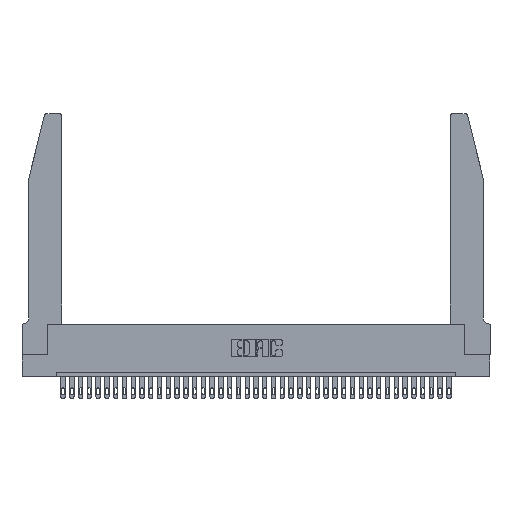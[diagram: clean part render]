
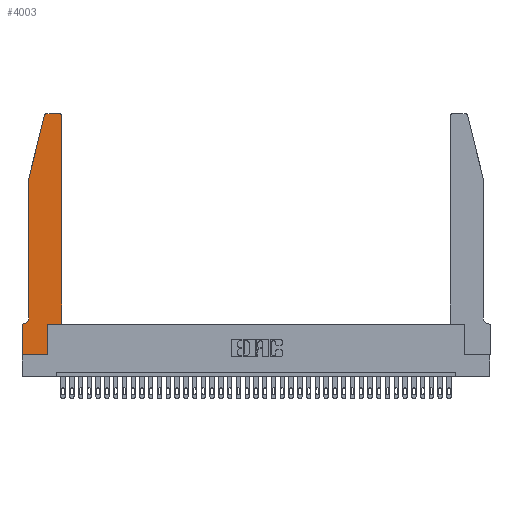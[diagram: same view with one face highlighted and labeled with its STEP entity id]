
A CAD part, top view. The second image highlights one B-rep face of the part: STEP entity #4003.
In plain terms, the highlighted planar face has unit normal (0, 0, 1).
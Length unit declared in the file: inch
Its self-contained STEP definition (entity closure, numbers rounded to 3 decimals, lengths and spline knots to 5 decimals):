
#663 = EDGE_CURVE ( 'NONE', #30695, #31927, #8686, .T. ) ;
#810 = FACE_OUTER_BOUND ( 'NONE', #34364, .T. ) ;
#1058 = ORIENTED_EDGE ( 'NONE', *, *, #20345, .T. ) ;
#1081 = CARTESIAN_POINT ( 'NONE',  ( 0.4505, 2.72, 0.37 ) ) ;
#1657 = CARTESIAN_POINT ( 'NONE',  ( 0.4505, 0.35, 0.37 ) ) ;
#1691 = DIRECTION ( 'NONE',  ( 1., 0., 0. ) ) ;
#2081 = VECTOR ( 'NONE', #19001, 39.37008 ) ;
#2313 = VERTEX_POINT ( 'NONE', #20618 ) ;
#2601 = CIRCLE ( 'NONE', #14978, 0.03 ) ;
#2822 = EDGE_CURVE ( 'NONE', #29767, #29390, #4620, .T. ) ;
#3044 = VECTOR ( 'NONE', #21404, 39.37008 ) ;
#3677 = AXIS2_PLACEMENT_3D ( 'NONE', #16455, #25176, #33824 ) ;
#3900 = CIRCLE ( 'NONE', #3677, 0.03 ) ;
#4003 = ADVANCED_FACE ( 'NONE', ( #810 ), #4917, .T. ) ;
#4620 = LINE ( 'NONE', #9189, #35060 ) ;
#4917 = PLANE ( 'NONE',  #35814 ) ;
#5079 = VECTOR ( 'NONE', #15449, 39.37008 ) ;
#5183 = DIRECTION ( 'NONE',  ( 0., -1., 0. ) ) ;
#5932 = VECTOR ( 'NONE', #5183, 39.37008 ) ;
#6243 = EDGE_CURVE ( 'NONE', #29390, #14842, #16583, .T. ) ;
#6562 = CARTESIAN_POINT ( 'NONE',  ( 0.284, 2.75, 0.37 ) ) ;
#6778 = ORIENTED_EDGE ( 'NONE', *, *, #32845, .T. ) ;
#6793 = VECTOR ( 'NONE', #25274, 39.37008 ) ;
#6817 = ORIENTED_EDGE ( 'NONE', *, *, #2822, .T. ) ;
#7348 = DIRECTION ( 'NONE',  ( -1., 0., 0. ) ) ;
#7484 = CARTESIAN_POINT ( 'NONE',  ( 0.2605, 2.75, 0.37 ) ) ;
#7898 = DIRECTION ( 'NONE',  ( 0., 0., 1. ) ) ;
#8686 = LINE ( 'NONE', #1657, #10536 ) ;
#9189 = CARTESIAN_POINT ( 'NONE',  ( 0.0755, 2., 0.37 ) ) ;
#9199 = VERTEX_POINT ( 'NONE', #22762 ) ;
#9320 = CARTESIAN_POINT ( 'NONE',  ( 0.0755, 0.35, 0.37 ) ) ;
#10508 = VERTEX_POINT ( 'NONE', #23438 ) ;
#10536 = VECTOR ( 'NONE', #34135, 39.37008 ) ;
#10606 = CARTESIAN_POINT ( 'NONE',  ( 0.4205, 2.75, 0.37 ) ) ;
#10871 = CARTESIAN_POINT ( 'NONE',  ( 0., 0.35, 0.37 ) ) ;
#12370 = CARTESIAN_POINT ( 'NONE',  ( 0.0755, 0.42, 0.37 ) ) ;
#13164 = CARTESIAN_POINT ( 'NONE',  ( 0., 0., 0.37 ) ) ;
#13927 = CARTESIAN_POINT ( 'NONE',  ( 0.4505, 0.35, 0.37 ) ) ;
#14587 = ORIENTED_EDGE ( 'NONE', *, *, #22725, .T. ) ;
#14842 = VERTEX_POINT ( 'NONE', #12370 ) ;
#14978 = AXIS2_PLACEMENT_3D ( 'NONE', #21487, #36275, #33474 ) ;
#15449 = DIRECTION ( 'NONE',  ( 1., 0., 0. ) ) ;
#16076 = CARTESIAN_POINT ( 'NONE',  ( 0., 0., 0.37 ) ) ;
#16382 = ORIENTED_EDGE ( 'NONE', *, *, #663, .T. ) ;
#16436 = CARTESIAN_POINT ( 'NONE',  ( 0.0055, 0.42, 0.37 ) ) ;
#16455 = CARTESIAN_POINT ( 'NONE',  ( 0.284, 2.72, 0.37 ) ) ;
#16583 = LINE ( 'NONE', #36699, #5932 ) ;
#16997 = LINE ( 'NONE', #7484, #25711 ) ;
#17065 = LINE ( 'NONE', #21554, #5079 ) ;
#17126 = VERTEX_POINT ( 'NONE', #13164 ) ;
#17236 = ORIENTED_EDGE ( 'NONE', *, *, #33155, .T. ) ;
#18017 = CARTESIAN_POINT ( 'NONE',  ( 0.2865, 0.35, 0.37 ) ) ;
#18339 = DIRECTION ( 'NONE',  ( -0.239, -0.971, 0. ) ) ;
#19001 = DIRECTION ( 'NONE',  ( 0., -1., 0. ) ) ;
#19483 = ORIENTED_EDGE ( 'NONE', *, *, #6243, .T. ) ;
#19868 = CARTESIAN_POINT ( 'NONE',  ( 0.25487, 2.72718, 0.37 ) ) ;
#20345 = EDGE_CURVE ( 'NONE', #17126, #9199, #17065, .T. ) ;
#20618 = CARTESIAN_POINT ( 'NONE',  ( 0., 0.35, 0.37 ) ) ;
#21211 = ORIENTED_EDGE ( 'NONE', *, *, #29633, .T. ) ;
#21277 = CARTESIAN_POINT ( 'NONE',  ( 0.4505, 0.35, 0.37 ) ) ;
#21404 = DIRECTION ( 'NONE',  ( 1., 0., 0. ) ) ;
#21454 = LINE ( 'NONE', #16076, #2081 ) ;
#21487 = CARTESIAN_POINT ( 'NONE',  ( 0.4205, 2.72, 0.37 ) ) ;
#21554 = CARTESIAN_POINT ( 'NONE',  ( 0., 0., 0.37 ) ) ;
#21555 = ORIENTED_EDGE ( 'NONE', *, *, #33803, .T. ) ;
#22725 = EDGE_CURVE ( 'NONE', #33536, #30695, #24737, .T. ) ;
#22762 = CARTESIAN_POINT ( 'NONE',  ( 0.2865, 0., 0.37 ) ) ;
#22774 = AXIS2_PLACEMENT_3D ( 'NONE', #16436, #34038, #31471 ) ;
#23438 = CARTESIAN_POINT ( 'NONE',  ( 0.0055, 0.35, 0.37 ) ) ;
#23703 = EDGE_CURVE ( 'NONE', #30499, #29767, #3900, .T. ) ;
#24145 = EDGE_CURVE ( 'NONE', #10508, #2313, #25940, .T. ) ;
#24269 = DIRECTION ( 'NONE',  ( -1., 0., 0. ) ) ;
#24737 = LINE ( 'NONE', #21277, #3044 ) ;
#25023 = VECTOR ( 'NONE', #24269, 39.37008 ) ;
#25176 = DIRECTION ( 'NONE',  ( 0., 0., 1. ) ) ;
#25274 = DIRECTION ( 'NONE',  ( 0., 1., 0. ) ) ;
#25459 = ORIENTED_EDGE ( 'NONE', *, *, #23703, .T. ) ;
#25711 = VECTOR ( 'NONE', #7348, 39.37008 ) ;
#25940 = LINE ( 'NONE', #9320, #25023 ) ;
#27345 = EDGE_CURVE ( 'NONE', #9199, #33536, #33991, .T. ) ;
#27359 = VERTEX_POINT ( 'NONE', #10606 ) ;
#28711 = ORIENTED_EDGE ( 'NONE', *, *, #24145, .T. ) ;
#29390 = VERTEX_POINT ( 'NONE', #32794 ) ;
#29633 = EDGE_CURVE ( 'NONE', #14842, #10508, #30134, .T. ) ;
#29767 = VERTEX_POINT ( 'NONE', #19868 ) ;
#30134 = CIRCLE ( 'NONE', #22774, 0.07 ) ;
#30499 = VERTEX_POINT ( 'NONE', #6562 ) ;
#30695 = VERTEX_POINT ( 'NONE', #13927 ) ;
#31471 = DIRECTION ( 'NONE',  ( -1., 0., 0. ) ) ;
#31927 = VERTEX_POINT ( 'NONE', #1081 ) ;
#32794 = CARTESIAN_POINT ( 'NONE',  ( 0.0755, 2., 0.37 ) ) ;
#32845 = EDGE_CURVE ( 'NONE', #27359, #30499, #16997, .T. ) ;
#33155 = EDGE_CURVE ( 'NONE', #31927, #27359, #2601, .T. ) ;
#33369 = ORIENTED_EDGE ( 'NONE', *, *, #27345, .T. ) ;
#33474 = DIRECTION ( 'NONE',  ( 1., 0., 0. ) ) ;
#33536 = VERTEX_POINT ( 'NONE', #18017 ) ;
#33803 = EDGE_CURVE ( 'NONE', #2313, #17126, #21454, .T. ) ;
#33824 = DIRECTION ( 'NONE',  ( 1., 0., 0. ) ) ;
#33991 = LINE ( 'NONE', #34556, #6793 ) ;
#34038 = DIRECTION ( 'NONE',  ( 0., 0., -1. ) ) ;
#34135 = DIRECTION ( 'NONE',  ( 0., 1., 0. ) ) ;
#34364 = EDGE_LOOP ( 'NONE', ( #6778, #25459, #6817, #19483, #21211, #28711, #21555, #1058, #33369, #14587, #16382, #17236 ) ) ;
#34556 = CARTESIAN_POINT ( 'NONE',  ( 0.2865, 0.35, 0.37 ) ) ;
#35060 = VECTOR ( 'NONE', #18339, 39.37008 ) ;
#35814 = AXIS2_PLACEMENT_3D ( 'NONE', #10871, #7898, #1691 ) ;
#36275 = DIRECTION ( 'NONE',  ( 0., 0., 1. ) ) ;
#36699 = CARTESIAN_POINT ( 'NONE',  ( 0.0755, 2., 0.37 ) ) ;
